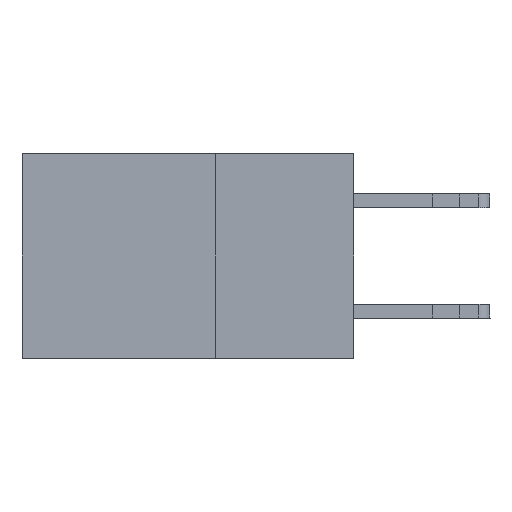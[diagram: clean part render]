
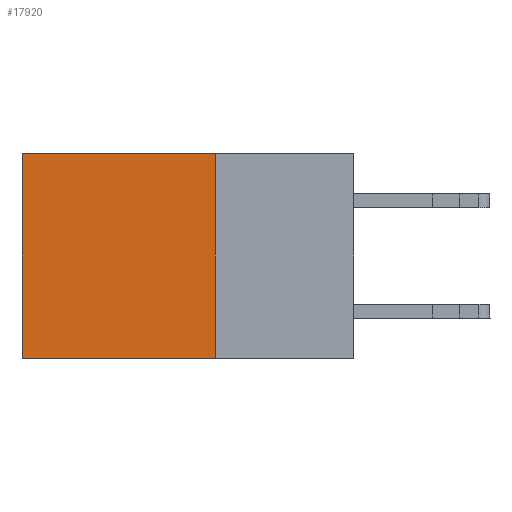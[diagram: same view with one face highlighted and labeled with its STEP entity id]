
A CAD part, left-side view. The second image highlights one B-rep face of the part: STEP entity #17920.
In plain terms, the highlighted planar face has unit normal (-1, 0, 0).
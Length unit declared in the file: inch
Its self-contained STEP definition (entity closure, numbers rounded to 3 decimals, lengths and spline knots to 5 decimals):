
#168 = LINE ( 'NONE', #22370, #24256 ) ;
#934 = DIRECTION ( 'NONE',  ( 0., 1., 0. ) ) ;
#1171 = AXIS2_PLACEMENT_3D ( 'NONE', #16485, #4051, #20966 ) ;
#1441 = ORIENTED_EDGE ( 'NONE', *, *, #11190, .F. ) ;
#4051 = DIRECTION ( 'NONE',  ( 1., 0., 0. ) ) ;
#4413 = CARTESIAN_POINT ( 'NONE',  ( 0.2875, 0.6, 0. ) ) ;
#5036 = CARTESIAN_POINT ( 'NONE',  ( 0.2875, 0.25, 0. ) ) ;
#5567 = EDGE_LOOP ( 'NONE', ( #22368, #14492, #1441, #6916 ) ) ;
#6369 = DIRECTION ( 'NONE',  ( 0., 1., 0. ) ) ;
#6814 = VERTEX_POINT ( 'NONE', #6854 ) ;
#6854 = CARTESIAN_POINT ( 'NONE',  ( 0.2875, 0.25, -0.37 ) ) ;
#6916 = ORIENTED_EDGE ( 'NONE', *, *, #20489, .T. ) ;
#7935 = VERTEX_POINT ( 'NONE', #19345 ) ;
#9090 = VECTOR ( 'NONE', #6369, 39.37008 ) ;
#10399 = LINE ( 'NONE', #5036, #17883 ) ;
#10786 = CARTESIAN_POINT ( 'NONE',  ( 0.2875, 0.25, 0. ) ) ;
#11190 = EDGE_CURVE ( 'NONE', #21657, #6814, #23185, .T. ) ;
#12114 = EDGE_CURVE ( 'NONE', #6814, #7935, #14579, .T. ) ;
#12453 = FACE_OUTER_BOUND ( 'NONE', #5567, .T. ) ;
#12554 = PLANE ( 'NONE',  #1171 ) ;
#14492 = ORIENTED_EDGE ( 'NONE', *, *, #12114, .F. ) ;
#14579 = LINE ( 'NONE', #21200, #9090 ) ;
#16485 = CARTESIAN_POINT ( 'NONE',  ( 0.2875, 0.25, 0. ) ) ;
#17883 = VECTOR ( 'NONE', #934, 39.37008 ) ;
#17920 = ADVANCED_FACE ( 'NONE', ( #12453 ), #12554, .F. ) ;
#19345 = CARTESIAN_POINT ( 'NONE',  ( 0.2875, 0.6, -0.37 ) ) ;
#20489 = EDGE_CURVE ( 'NONE', #21657, #22315, #10399, .T. ) ;
#20966 = DIRECTION ( 'NONE',  ( 0., 0., -1. ) ) ;
#21200 = CARTESIAN_POINT ( 'NONE',  ( 0.2875, 0.25, -0.37 ) ) ;
#21657 = VERTEX_POINT ( 'NONE', #10786 ) ;
#22315 = VERTEX_POINT ( 'NONE', #4413 ) ;
#22368 = ORIENTED_EDGE ( 'NONE', *, *, #26876, .T. ) ;
#22370 = CARTESIAN_POINT ( 'NONE',  ( 0.2875, 0.6, 0. ) ) ;
#22629 = DIRECTION ( 'NONE',  ( 0., 0., -1. ) ) ;
#23185 = LINE ( 'NONE', #26885, #25105 ) ;
#24256 = VECTOR ( 'NONE', #26716, 39.37008 ) ;
#25105 = VECTOR ( 'NONE', #22629, 39.37008 ) ;
#26716 = DIRECTION ( 'NONE',  ( 0., 0., -1. ) ) ;
#26876 = EDGE_CURVE ( 'NONE', #22315, #7935, #168, .T. ) ;
#26885 = CARTESIAN_POINT ( 'NONE',  ( 0.2875, 0.25, 0. ) ) ;
